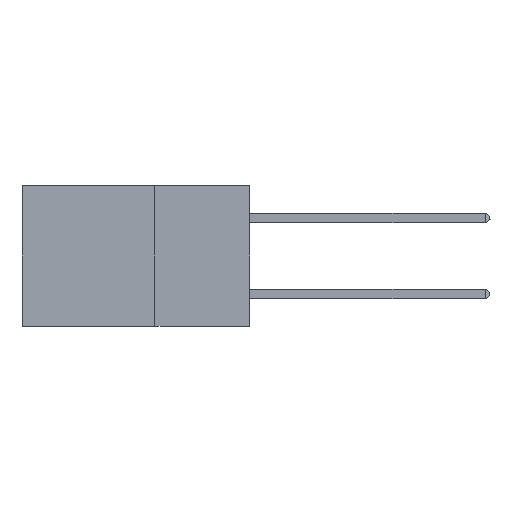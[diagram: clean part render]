
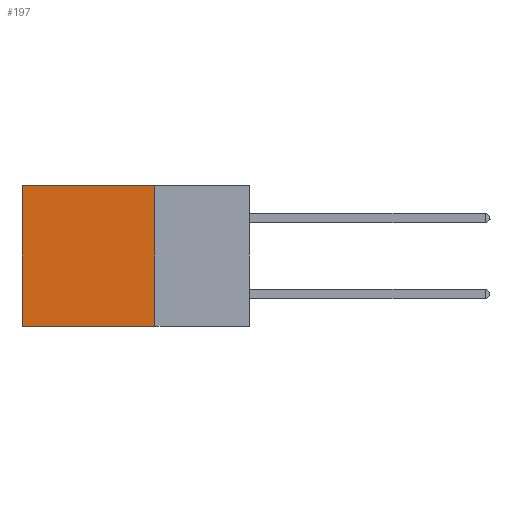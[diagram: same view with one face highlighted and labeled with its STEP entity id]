
A CAD part, left-side view. The second image highlights one B-rep face of the part: STEP entity #197.
In plain terms, the highlighted planar face has unit normal (-1, 0, 0).
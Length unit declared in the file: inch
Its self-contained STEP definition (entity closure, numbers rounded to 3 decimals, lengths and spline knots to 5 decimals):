
#197 = ADVANCED_FACE ( 'NONE', ( #27625 ), #5797, .F. ) ;
#1125 = EDGE_CURVE ( 'NONE', #5082, #17401, #16336, .T. ) ;
#1168 = VECTOR ( 'NONE', #4223, 39.37008 ) ;
#1954 = CARTESIAN_POINT ( 'NONE',  ( 0.2875, 0.25, -0.37 ) ) ;
#3407 = DIRECTION ( 'NONE',  ( 0., 0., -1. ) ) ;
#3668 = DIRECTION ( 'NONE',  ( 0., 0., -1. ) ) ;
#4223 = DIRECTION ( 'NONE',  ( 0., 1., 0. ) ) ;
#4380 = CARTESIAN_POINT ( 'NONE',  ( 0.2875, 0.25, 0. ) ) ;
#4389 = EDGE_CURVE ( 'NONE', #5082, #28086, #29443, .T. ) ;
#4407 = VERTEX_POINT ( 'NONE', #7782 ) ;
#4419 = CARTESIAN_POINT ( 'NONE',  ( 0.2875, 0.6, 0. ) ) ;
#5082 = VERTEX_POINT ( 'NONE', #14523 ) ;
#5797 = PLANE ( 'NONE',  #27536 ) ;
#7611 = CARTESIAN_POINT ( 'NONE',  ( 0.2875, 0.25, 0. ) ) ;
#7782 = CARTESIAN_POINT ( 'NONE',  ( 0.2875, 0.6, -0.37 ) ) ;
#9925 = ORIENTED_EDGE ( 'NONE', *, *, #13444, .F. ) ;
#11068 = CARTESIAN_POINT ( 'NONE',  ( 0.2875, 0.25, -0.37 ) ) ;
#13444 = EDGE_CURVE ( 'NONE', #28086, #4407, #17064, .T. ) ;
#14523 = CARTESIAN_POINT ( 'NONE',  ( 0.2875, 0.25, 0. ) ) ;
#14623 = VECTOR ( 'NONE', #29605, 39.37008 ) ;
#15519 = CARTESIAN_POINT ( 'NONE',  ( 0.2875, 0.25, 0. ) ) ;
#15937 = LINE ( 'NONE', #26124, #24937 ) ;
#15967 = EDGE_LOOP ( 'NONE', ( #30124, #9925, #21432, #23136 ) ) ;
#16336 = LINE ( 'NONE', #4380, #1168 ) ;
#17064 = LINE ( 'NONE', #11068, #18527 ) ;
#17401 = VERTEX_POINT ( 'NONE', #4419 ) ;
#18527 = VECTOR ( 'NONE', #26457, 39.37008 ) ;
#21432 = ORIENTED_EDGE ( 'NONE', *, *, #4389, .F. ) ;
#23136 = ORIENTED_EDGE ( 'NONE', *, *, #1125, .T. ) ;
#24937 = VECTOR ( 'NONE', #3668, 39.37008 ) ;
#25227 = DIRECTION ( 'NONE',  ( 1., 0., 0. ) ) ;
#26124 = CARTESIAN_POINT ( 'NONE',  ( 0.2875, 0.6, 0. ) ) ;
#26457 = DIRECTION ( 'NONE',  ( 0., 1., 0. ) ) ;
#27536 = AXIS2_PLACEMENT_3D ( 'NONE', #15519, #25227, #3407 ) ;
#27625 = FACE_OUTER_BOUND ( 'NONE', #15967, .T. ) ;
#28086 = VERTEX_POINT ( 'NONE', #1954 ) ;
#29443 = LINE ( 'NONE', #7611, #14623 ) ;
#29605 = DIRECTION ( 'NONE',  ( 0., 0., -1. ) ) ;
#30124 = ORIENTED_EDGE ( 'NONE', *, *, #30729, .T. ) ;
#30729 = EDGE_CURVE ( 'NONE', #17401, #4407, #15937, .T. ) ;
